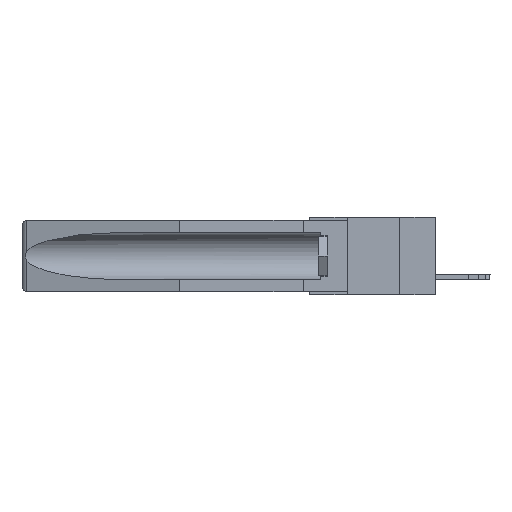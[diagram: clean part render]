
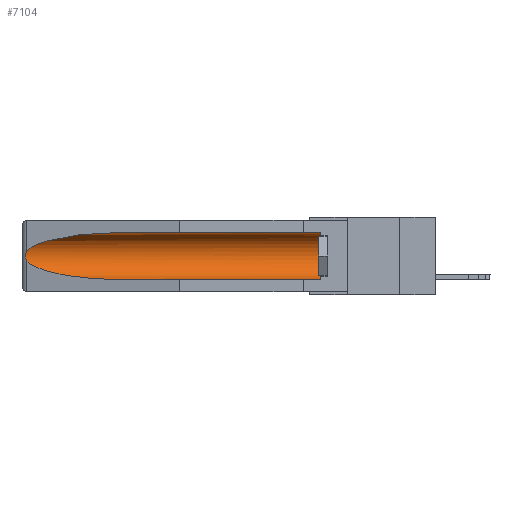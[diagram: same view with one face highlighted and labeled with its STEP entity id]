
A CAD part, left-side view. The second image highlights one B-rep face of the part: STEP entity #7104.
In plain terms, the highlighted cylindrical face has radius 2.857 mm (diameter 5.715 mm), a partial arc.
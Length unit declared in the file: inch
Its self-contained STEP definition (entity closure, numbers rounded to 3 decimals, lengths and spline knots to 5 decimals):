
#285 = CARTESIAN_POINT ( 'NONE',  ( 0.26537, 1.52718, -0.19328 ) ) ;
#1012 = LINE ( 'NONE', #4358, #18655 ) ;
#1100 = DIRECTION ( 'NONE',  ( 0., 1., 0. ) ) ;
#1450 = CYLINDRICAL_SURFACE ( 'NONE', #9738, 0.1125 ) ;
#1868 = CARTESIAN_POINT ( 'NONE',  ( 0.155, 1.07973, -0.059 ) ) ;
#1917 = CARTESIAN_POINT ( 'NONE',  ( 0.2675, 1.53308, -0.17534 ) ) ;
#2397 = EDGE_CURVE ( 'NONE', #12743, #5913, #1012, .T. ) ;
#2997 = EDGE_CURVE ( 'NONE', #4796, #5913, #4435, .T. ) ;
#3184 = CARTESIAN_POINT ( 'NONE',  ( 0.26597, 1.52961, -0.15275 ) ) ;
#3359 = CARTESIAN_POINT ( 'NONE',  ( 0.155, 0.126, -0.1715 ) ) ;
#3528 = ORIENTED_EDGE ( 'NONE', *, *, #2397, .F. ) ;
#3551 = VECTOR ( 'NONE', #1100, 39.37008 ) ;
#3552 = CARTESIAN_POINT ( 'NONE',  ( 0.26537, 1.52718, -0.19328 ) ) ;
#3802 = LINE ( 'NONE', #10860, #3551 ) ;
#4358 = CARTESIAN_POINT ( 'NONE',  ( 0.155, -0.30754, -0.284 ) ) ;
#4435 =( BOUNDED_CURVE ( )  B_SPLINE_CURVE ( 3, ( #3552, #18849, #4445, #15626 ),
 .UNSPECIFIED., .F., .F. ) 
 B_SPLINE_CURVE_WITH_KNOTS ( ( 4, 4 ),
 ( 0.1948, 1.5708 ),
 .UNSPECIFIED. ) 
 CURVE ( )  GEOMETRIC_REPRESENTATION_ITEM ( )  RATIONAL_B_SPLINE_CURVE ( ( 1., 0.848, 0.848, 1. ) ) 
 REPRESENTATION_ITEM ( '' )  );
#4445 = CARTESIAN_POINT ( 'NONE',  ( 0.21114, 1.30732, -0.284 ) ) ;
#4495 = CARTESIAN_POINT ( 'NONE',  ( 0.26537, 1.52718, -0.14972 ) ) ;
#4796 = VERTEX_POINT ( 'NONE', #285 ) ;
#5014 = ORIENTED_EDGE ( 'NONE', *, *, #2997, .T. ) ;
#5062 = DIRECTION ( 'NONE',  ( 0., 0., 1. ) ) ;
#5085 =( BOUNDED_CURVE ( )  B_SPLINE_CURVE ( 3, ( #14249, #15906, #14728, #19551 ),
 .UNSPECIFIED., .F., .F. ) 
 B_SPLINE_CURVE_WITH_KNOTS ( ( 4, 4 ),
 ( 4.71239, 6.08839 ),
 .UNSPECIFIED. ) 
 CURVE ( )  GEOMETRIC_REPRESENTATION_ITEM ( )  RATIONAL_B_SPLINE_CURVE ( ( 1., 0.848, 0.848, 1. ) ) 
 REPRESENTATION_ITEM ( '' )  );
#5440 = EDGE_CURVE ( 'NONE', #6972, #10012, #3802, .T. ) ;
#5675 = EDGE_CURVE ( 'NONE', #12743, #6972, #6604, .T. ) ;
#5913 = VERTEX_POINT ( 'NONE', #8733 ) ;
#6448 = CARTESIAN_POINT ( 'NONE',  ( 0.2673, 1.53269, -0.17917 ) ) ;
#6604 = CIRCLE ( 'NONE', #13102, 0.1125 ) ;
#6733 = CARTESIAN_POINT ( 'NONE',  ( 0.26537, 1.52718, -0.19328 ) ) ;
#6972 = VERTEX_POINT ( 'NONE', #16903 ) ;
#7104 = ADVANCED_FACE ( 'NONE', ( #12812 ), #1450, .F. ) ;
#7409 = ORIENTED_EDGE ( 'NONE', *, *, #5675, .T. ) ;
#8367 = CARTESIAN_POINT ( 'NONE',  ( 0.2675, 1.53308, -0.16763 ) ) ;
#8733 = CARTESIAN_POINT ( 'NONE',  ( 0.155, 1.07973, -0.284 ) ) ;
#9153 = DIRECTION ( 'NONE',  ( 0., 1., 0. ) ) ;
#9738 = AXIS2_PLACEMENT_3D ( 'NONE', #20272, #9153, #15730 ) ;
#10012 = VERTEX_POINT ( 'NONE', #1868 ) ;
#10472 = EDGE_CURVE ( 'NONE', #10012, #11988, #5085, .T. ) ;
#10860 = CARTESIAN_POINT ( 'NONE',  ( 0.155, -0.30754, -0.059 ) ) ;
#11264 = EDGE_LOOP ( 'NONE', ( #18320, #20415, #5014, #3528, #7409, #18508 ) ) ;
#11289 = CARTESIAN_POINT ( 'NONE',  ( 0.26597, 1.5296, -0.19026 ) ) ;
#11428 = CARTESIAN_POINT ( 'NONE',  ( 0.26655, 1.53094, -0.18657 ) ) ;
#11988 = VERTEX_POINT ( 'NONE', #4495 ) ;
#12743 = VERTEX_POINT ( 'NONE', #17694 ) ;
#12812 = FACE_OUTER_BOUND ( 'NONE', #11264, .T. ) ;
#13102 = AXIS2_PLACEMENT_3D ( 'NONE', #3359, #14701, #5062 ) ;
#13789 = DIRECTION ( 'NONE',  ( 0., 1., 0. ) ) ;
#14249 = CARTESIAN_POINT ( 'NONE',  ( 0.155, 1.07973, -0.059 ) ) ;
#14701 = DIRECTION ( 'NONE',  ( 0., -1., 0. ) ) ;
#14728 = CARTESIAN_POINT ( 'NONE',  ( 0.25451, 1.48313, -0.09465 ) ) ;
#15626 = CARTESIAN_POINT ( 'NONE',  ( 0.155, 1.07973, -0.284 ) ) ;
#15711 = CARTESIAN_POINT ( 'NONE',  ( 0.26654, 1.53092, -0.15636 ) ) ;
#15730 = DIRECTION ( 'NONE',  ( 0., 0., 1. ) ) ;
#15906 = CARTESIAN_POINT ( 'NONE',  ( 0.21114, 1.30732, -0.059 ) ) ;
#16075 = CARTESIAN_POINT ( 'NONE',  ( 0.2673, 1.5327, -0.16383 ) ) ;
#16302 = B_SPLINE_CURVE_WITH_KNOTS ( 'NONE', 3,
 ( #17538, #3184, #15711, #16075, #8367, #1917, #6448, #11428, #11289, #6733 ),
 .UNSPECIFIED., .F., .F.,
 ( 4, 2, 2, 2, 4 ),
 ( 0., 0.00029, 0.00058, 0.00087, 0.00117 ),
 .UNSPECIFIED. ) ;
#16903 = CARTESIAN_POINT ( 'NONE',  ( 0.155, 0.126, -0.059 ) ) ;
#17538 = CARTESIAN_POINT ( 'NONE',  ( 0.26537, 1.52718, -0.14972 ) ) ;
#17694 = CARTESIAN_POINT ( 'NONE',  ( 0.155, 0.126, -0.284 ) ) ;
#18176 = EDGE_CURVE ( 'NONE', #11988, #4796, #16302, .T. ) ;
#18320 = ORIENTED_EDGE ( 'NONE', *, *, #10472, .T. ) ;
#18508 = ORIENTED_EDGE ( 'NONE', *, *, #5440, .T. ) ;
#18655 = VECTOR ( 'NONE', #13789, 39.37008 ) ;
#18849 = CARTESIAN_POINT ( 'NONE',  ( 0.25451, 1.48313, -0.24835 ) ) ;
#19551 = CARTESIAN_POINT ( 'NONE',  ( 0.26537, 1.52718, -0.14972 ) ) ;
#20272 = CARTESIAN_POINT ( 'NONE',  ( 0.155, -0.30754, -0.1715 ) ) ;
#20415 = ORIENTED_EDGE ( 'NONE', *, *, #18176, .T. ) ;
